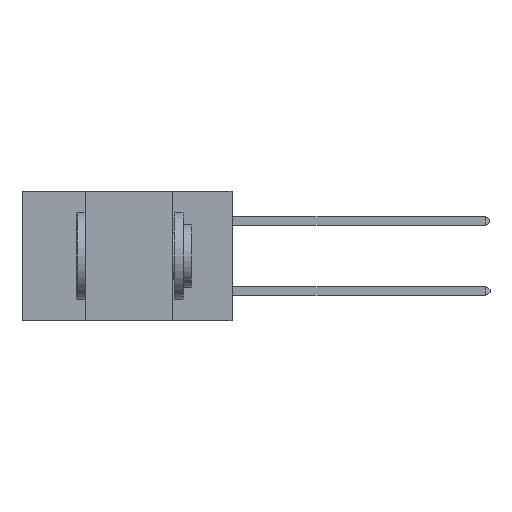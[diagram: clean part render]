
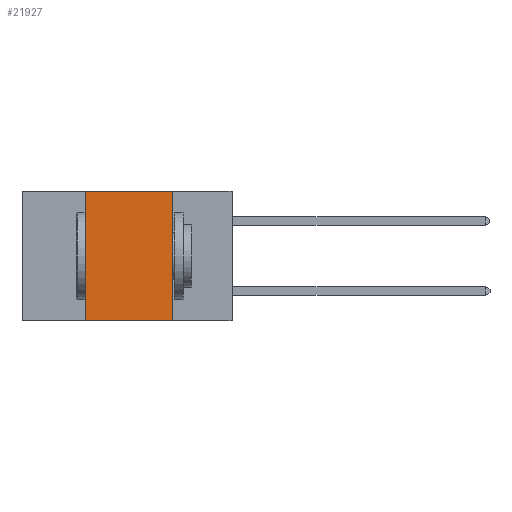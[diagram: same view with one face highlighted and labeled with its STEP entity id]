
A CAD part, left-side view. The second image highlights one B-rep face of the part: STEP entity #21927.
In plain terms, the highlighted planar face has unit normal (-1, 0, 0).
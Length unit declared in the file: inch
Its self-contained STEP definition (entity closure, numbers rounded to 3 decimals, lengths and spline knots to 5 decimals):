
#609 = VECTOR ( 'NONE', #16300, 39.37008 ) ;
#1360 = PLANE ( 'NONE',  #12750 ) ;
#2377 = CARTESIAN_POINT ( 'NONE',  ( 0., 0.6, 0. ) ) ;
#3351 = CARTESIAN_POINT ( 'NONE',  ( 0., 0.6, 0. ) ) ;
#3355 = CARTESIAN_POINT ( 'NONE',  ( 0., 0.17, -0.37 ) ) ;
#4816 = CARTESIAN_POINT ( 'NONE',  ( 0., 0.42, 0. ) ) ;
#4964 = CARTESIAN_POINT ( 'NONE',  ( 0., 0.6, -0.37 ) ) ;
#5279 = DIRECTION ( 'NONE',  ( 0., 0., 1. ) ) ;
#5407 = DIRECTION ( 'NONE',  ( 0., -1., 0. ) ) ;
#6626 = CARTESIAN_POINT ( 'NONE',  ( 0., 0.17, 0. ) ) ;
#7060 = EDGE_CURVE ( 'NONE', #21839, #21608, #15293, .T. ) ;
#8535 = CARTESIAN_POINT ( 'NONE',  ( 0., 0.42, 0. ) ) ;
#9192 = ORIENTED_EDGE ( 'NONE', *, *, #15949, .F. ) ;
#10130 = VECTOR ( 'NONE', #5407, 39.37008 ) ;
#10288 = LINE ( 'NONE', #4964, #12728 ) ;
#10551 = CARTESIAN_POINT ( 'NONE',  ( 0., 0.42, -0.37 ) ) ;
#10661 = DIRECTION ( 'NONE',  ( 0., -1., 0. ) ) ;
#11919 = ORIENTED_EDGE ( 'NONE', *, *, #7060, .F. ) ;
#12497 = EDGE_CURVE ( 'NONE', #18589, #20701, #10288, .T. ) ;
#12728 = VECTOR ( 'NONE', #10661, 39.37008 ) ;
#12750 = AXIS2_PLACEMENT_3D ( 'NONE', #3351, #12885, #15249 ) ;
#12885 = DIRECTION ( 'NONE',  ( 1., 0., 0. ) ) ;
#12986 = CARTESIAN_POINT ( 'NONE',  ( 0., 0.17, 0. ) ) ;
#13515 = EDGE_CURVE ( 'NONE', #18589, #21839, #20900, .T. ) ;
#15249 = DIRECTION ( 'NONE',  ( 0., 0., -1. ) ) ;
#15293 = LINE ( 'NONE', #2377, #10130 ) ;
#15900 = FACE_OUTER_BOUND ( 'NONE', #22011, .T. ) ;
#15949 = EDGE_CURVE ( 'NONE', #21608, #20701, #24771, .T. ) ;
#16300 = DIRECTION ( 'NONE',  ( 0., 0., -1. ) ) ;
#17222 = VECTOR ( 'NONE', #5279, 39.37008 ) ;
#18589 = VERTEX_POINT ( 'NONE', #10551 ) ;
#20701 = VERTEX_POINT ( 'NONE', #3355 ) ;
#20900 = LINE ( 'NONE', #4816, #17222 ) ;
#21241 = ORIENTED_EDGE ( 'NONE', *, *, #12497, .T. ) ;
#21608 = VERTEX_POINT ( 'NONE', #12986 ) ;
#21839 = VERTEX_POINT ( 'NONE', #8535 ) ;
#21927 = ADVANCED_FACE ( 'NONE', ( #15900 ), #1360, .F. ) ;
#22011 = EDGE_LOOP ( 'NONE', ( #9192, #11919, #23901, #21241 ) ) ;
#23901 = ORIENTED_EDGE ( 'NONE', *, *, #13515, .F. ) ;
#24771 = LINE ( 'NONE', #6626, #609 ) ;
